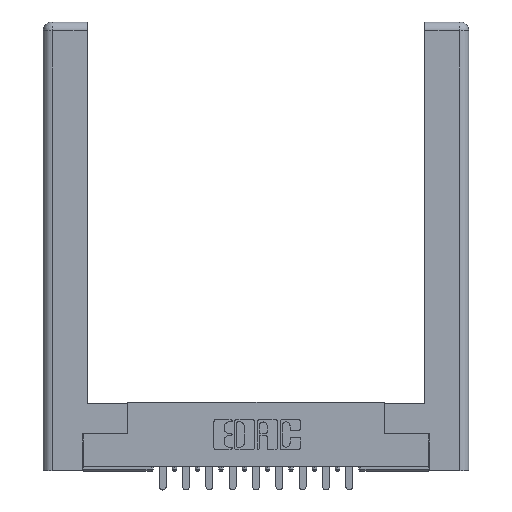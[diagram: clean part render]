
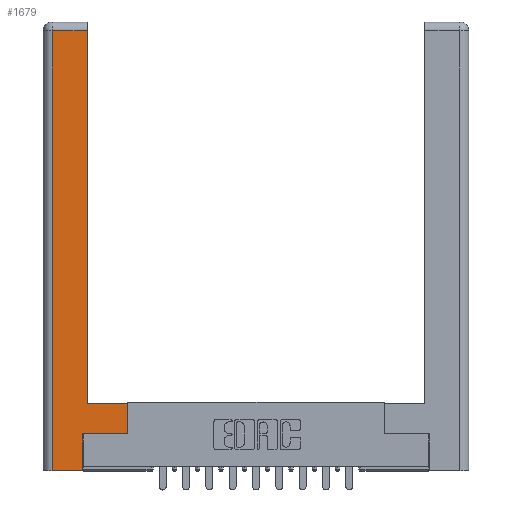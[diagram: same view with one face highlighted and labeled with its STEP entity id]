
A CAD part, top view. The second image highlights one B-rep face of the part: STEP entity #1679.
In plain terms, the highlighted planar face has unit normal (0, 0, 1).
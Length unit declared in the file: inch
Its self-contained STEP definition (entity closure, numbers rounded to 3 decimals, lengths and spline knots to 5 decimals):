
#481 = VECTOR ( 'NONE', #6628, 39.37008 ) ;
#692 = DIRECTION ( 'NONE',  ( 1., 0., 0. ) ) ;
#693 = ORIENTED_EDGE ( 'NONE', *, *, #11149, .T. ) ;
#1543 = FACE_OUTER_BOUND ( 'NONE', #2656, .T. ) ;
#1679 = ADVANCED_FACE ( 'NONE', ( #1543 ), #11482, .F. ) ;
#1796 = VECTOR ( 'NONE', #1959, 39.37008 ) ;
#1959 = DIRECTION ( 'NONE',  ( 0., 1., 0. ) ) ;
#2007 = VECTOR ( 'NONE', #14033, 39.37008 ) ;
#2044 = CARTESIAN_POINT ( 'NONE',  ( 0.295, 0.45, 0. ) ) ;
#2656 = EDGE_LOOP ( 'NONE', ( #5147, #4757, #16193, #11634, #14414, #3092, #693, #4192 ) ) ;
#2679 = VECTOR ( 'NONE', #13424, 39.37008 ) ;
#3092 = ORIENTED_EDGE ( 'NONE', *, *, #12209, .T. ) ;
#3243 = EDGE_CURVE ( 'NONE', #8894, #11528, #9391, .T. ) ;
#3848 = VERTEX_POINT ( 'NONE', #14754 ) ;
#3980 = DIRECTION ( 'NONE',  ( 0., 0., -1. ) ) ;
#4131 = VECTOR ( 'NONE', #7579, 39.37008 ) ;
#4192 = ORIENTED_EDGE ( 'NONE', *, *, #11893, .T. ) ;
#4229 = CARTESIAN_POINT ( 'NONE',  ( 0.0615, 2.94, 0. ) ) ;
#4234 = CARTESIAN_POINT ( 'NONE',  ( 0.295, 2.94, 0. ) ) ;
#4401 = CARTESIAN_POINT ( 'NONE',  ( 0.265, 0., 0. ) ) ;
#4600 = LINE ( 'NONE', #7956, #2007 ) ;
#4757 = ORIENTED_EDGE ( 'NONE', *, *, #5111, .T. ) ;
#4803 = LINE ( 'NONE', #2044, #7368 ) ;
#4914 = LINE ( 'NONE', #7629, #4131 ) ;
#5111 = EDGE_CURVE ( 'NONE', #11528, #6632, #15395, .T. ) ;
#5139 = CARTESIAN_POINT ( 'NONE',  ( 0.265, 0., 0. ) ) ;
#5147 = ORIENTED_EDGE ( 'NONE', *, *, #3243, .T. ) ;
#5182 = CARTESIAN_POINT ( 'NONE',  ( 0.565, 0.45, 0. ) ) ;
#6204 = LINE ( 'NONE', #5182, #481 ) ;
#6426 = CARTESIAN_POINT ( 'NONE',  ( 0., 0., 0. ) ) ;
#6628 = DIRECTION ( 'NONE',  ( 0., 1., 0. ) ) ;
#6632 = VERTEX_POINT ( 'NONE', #11517 ) ;
#7001 = CARTESIAN_POINT ( 'NONE',  ( 0.265, 0.245, 0. ) ) ;
#7099 = CARTESIAN_POINT ( 'NONE',  ( 0.0615, 0., 0. ) ) ;
#7368 = VECTOR ( 'NONE', #13291, 39.37008 ) ;
#7579 = DIRECTION ( 'NONE',  ( 0., -1., 0. ) ) ;
#7629 = CARTESIAN_POINT ( 'NONE',  ( 0.0615, 0., 0. ) ) ;
#7705 = DIRECTION ( 'NONE',  ( -1., 0., 0. ) ) ;
#7956 = CARTESIAN_POINT ( 'NONE',  ( 0.565, 0.245, 0. ) ) ;
#8203 = EDGE_CURVE ( 'NONE', #6632, #9709, #4914, .T. ) ;
#8348 = VERTEX_POINT ( 'NONE', #15514 ) ;
#8894 = VERTEX_POINT ( 'NONE', #9986 ) ;
#9174 = VECTOR ( 'NONE', #692, 39.37008 ) ;
#9391 = LINE ( 'NONE', #13480, #2679 ) ;
#9709 = VERTEX_POINT ( 'NONE', #7099 ) ;
#9986 = CARTESIAN_POINT ( 'NONE',  ( 0.295, 0.45, 0. ) ) ;
#10358 = VERTEX_POINT ( 'NONE', #5139 ) ;
#10540 = LINE ( 'NONE', #4401, #9174 ) ;
#11149 = EDGE_CURVE ( 'NONE', #3848, #11939, #6204, .T. ) ;
#11384 = AXIS2_PLACEMENT_3D ( 'NONE', #6426, #3980, #7705 ) ;
#11482 = PLANE ( 'NONE',  #11384 ) ;
#11517 = CARTESIAN_POINT ( 'NONE',  ( 0.0615, 2.94, 0. ) ) ;
#11528 = VERTEX_POINT ( 'NONE', #4234 ) ;
#11634 = ORIENTED_EDGE ( 'NONE', *, *, #15125, .T. ) ;
#11893 = EDGE_CURVE ( 'NONE', #11939, #8894, #4803, .T. ) ;
#11939 = VERTEX_POINT ( 'NONE', #14869 ) ;
#12209 = EDGE_CURVE ( 'NONE', #8348, #3848, #4600, .T. ) ;
#13045 = EDGE_CURVE ( 'NONE', #10358, #8348, #13230, .T. ) ;
#13083 = DIRECTION ( 'NONE',  ( -1., 0., 0. ) ) ;
#13230 = LINE ( 'NONE', #7001, #1796 ) ;
#13291 = DIRECTION ( 'NONE',  ( -1., 0., 0. ) ) ;
#13424 = DIRECTION ( 'NONE',  ( 0., 1., 0. ) ) ;
#13480 = CARTESIAN_POINT ( 'NONE',  ( 0.295, 3., 0. ) ) ;
#14033 = DIRECTION ( 'NONE',  ( 1., 0., 0. ) ) ;
#14224 = VECTOR ( 'NONE', #13083, 39.37008 ) ;
#14414 = ORIENTED_EDGE ( 'NONE', *, *, #13045, .T. ) ;
#14754 = CARTESIAN_POINT ( 'NONE',  ( 0.565, 0.245, 0. ) ) ;
#14869 = CARTESIAN_POINT ( 'NONE',  ( 0.565, 0.45, 0. ) ) ;
#15125 = EDGE_CURVE ( 'NONE', #9709, #10358, #10540, .T. ) ;
#15395 = LINE ( 'NONE', #4229, #14224 ) ;
#15514 = CARTESIAN_POINT ( 'NONE',  ( 0.265, 0.245, 0. ) ) ;
#16193 = ORIENTED_EDGE ( 'NONE', *, *, #8203, .T. ) ;
